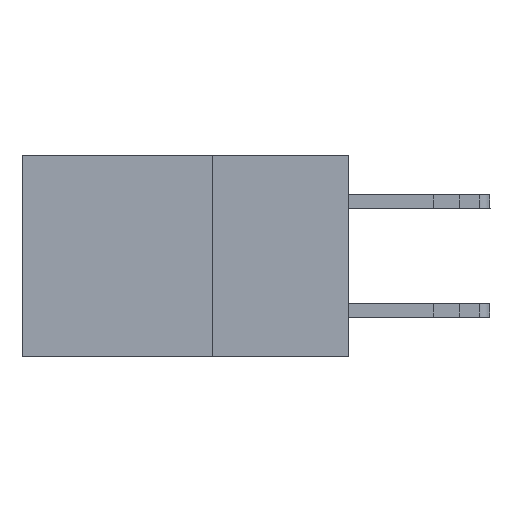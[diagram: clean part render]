
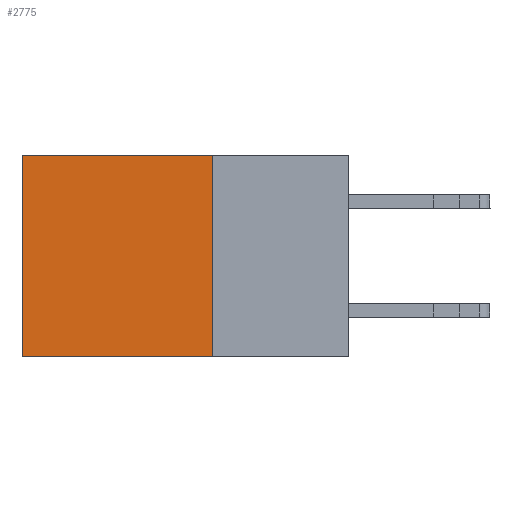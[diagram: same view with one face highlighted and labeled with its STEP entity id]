
A CAD part, left-side view. The second image highlights one B-rep face of the part: STEP entity #2775.
In plain terms, the highlighted planar face has unit normal (-1, 0, 0).
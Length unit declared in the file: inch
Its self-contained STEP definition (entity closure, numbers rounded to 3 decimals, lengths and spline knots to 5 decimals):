
#1694 = CARTESIAN_POINT ( 'NONE',  ( 0.298, 0.25, -0.37 ) ) ;
#2138 = DIRECTION ( 'NONE',  ( 1., 0., 0. ) ) ;
#2626 = VECTOR ( 'NONE', #8905, 39.37008 ) ;
#2775 = ADVANCED_FACE ( 'NONE', ( #12179 ), #3129, .F. ) ;
#3129 = PLANE ( 'NONE',  #8282 ) ;
#3960 = DIRECTION ( 'NONE',  ( 0., 0., -1. ) ) ;
#4030 = DIRECTION ( 'NONE',  ( 0., 1., 0. ) ) ;
#4380 = CARTESIAN_POINT ( 'NONE',  ( 0.298, 0.25, 0. ) ) ;
#5272 = VERTEX_POINT ( 'NONE', #4380 ) ;
#5882 = CARTESIAN_POINT ( 'NONE',  ( 0.298, 0.25, 0. ) ) ;
#6003 = VECTOR ( 'NONE', #3960, 39.37008 ) ;
#6125 = EDGE_CURVE ( 'NONE', #9460, #6916, #7554, .T. ) ;
#6165 = DIRECTION ( 'NONE',  ( 0., 0., -1. ) ) ;
#6176 = ORIENTED_EDGE ( 'NONE', *, *, #6125, .F. ) ;
#6916 = VERTEX_POINT ( 'NONE', #11308 ) ;
#6939 = LINE ( 'NONE', #13013, #6003 ) ;
#7159 = CARTESIAN_POINT ( 'NONE',  ( 0.298, 0.25, 0. ) ) ;
#7554 = LINE ( 'NONE', #10740, #7664 ) ;
#7652 = EDGE_CURVE ( 'NONE', #10553, #6916, #6939, .T. ) ;
#7664 = VECTOR ( 'NONE', #12585, 39.37008 ) ;
#8282 = AXIS2_PLACEMENT_3D ( 'NONE', #7159, #2138, #6165 ) ;
#8905 = DIRECTION ( 'NONE',  ( 0., 0., -1. ) ) ;
#9113 = CARTESIAN_POINT ( 'NONE',  ( 0.298, 0.25, 0. ) ) ;
#9233 = ORIENTED_EDGE ( 'NONE', *, *, #11707, .T. ) ;
#9460 = VERTEX_POINT ( 'NONE', #1694 ) ;
#10038 = LINE ( 'NONE', #9113, #10618 ) ;
#10553 = VERTEX_POINT ( 'NONE', #12824 ) ;
#10618 = VECTOR ( 'NONE', #4030, 39.37008 ) ;
#10740 = CARTESIAN_POINT ( 'NONE',  ( 0.298, 0.25, -0.37 ) ) ;
#11091 = EDGE_LOOP ( 'NONE', ( #12434, #6176, #12624, #9233 ) ) ;
#11097 = LINE ( 'NONE', #5882, #2626 ) ;
#11308 = CARTESIAN_POINT ( 'NONE',  ( 0.298, 0.6, -0.37 ) ) ;
#11707 = EDGE_CURVE ( 'NONE', #5272, #10553, #10038, .T. ) ;
#12179 = FACE_OUTER_BOUND ( 'NONE', #11091, .T. ) ;
#12184 = EDGE_CURVE ( 'NONE', #5272, #9460, #11097, .T. ) ;
#12434 = ORIENTED_EDGE ( 'NONE', *, *, #7652, .T. ) ;
#12585 = DIRECTION ( 'NONE',  ( 0., 1., 0. ) ) ;
#12624 = ORIENTED_EDGE ( 'NONE', *, *, #12184, .F. ) ;
#12824 = CARTESIAN_POINT ( 'NONE',  ( 0.298, 0.6, 0. ) ) ;
#13013 = CARTESIAN_POINT ( 'NONE',  ( 0.298, 0.6, 0. ) ) ;
